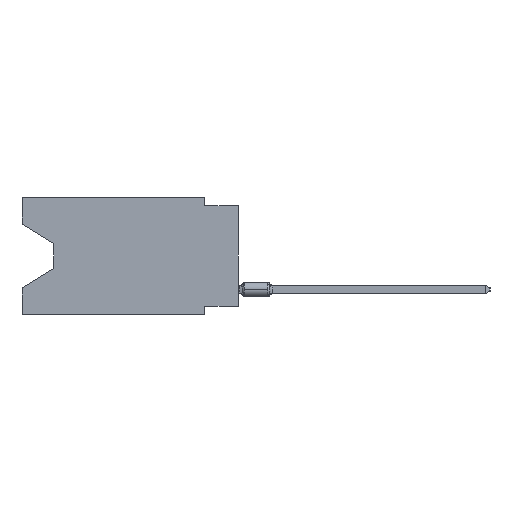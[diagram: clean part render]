
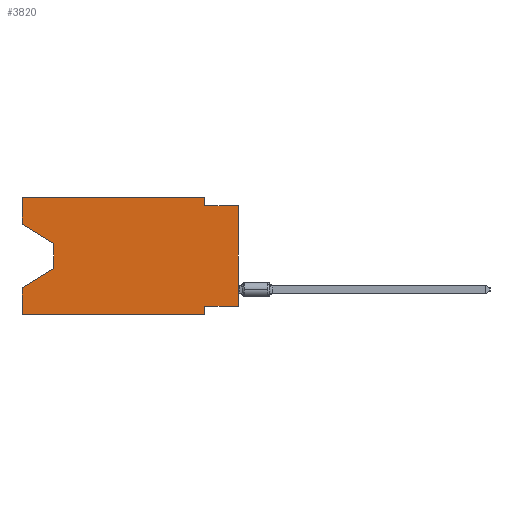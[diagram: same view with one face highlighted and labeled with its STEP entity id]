
A CAD part, left-side view. The second image highlights one B-rep face of the part: STEP entity #3820.
In plain terms, the highlighted planar face has unit normal (-1, 0, 0).
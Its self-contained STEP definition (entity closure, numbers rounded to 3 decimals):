
#179 = EDGE_CURVE ( 'NONE', #42953, #15369, #29749, .T. ) ;
#418 = CARTESIAN_POINT ( 'NONE',  ( 0., 16.383, 0. ) ) ;
#1485 = FACE_OUTER_BOUND ( 'NONE', #47448, .T. ) ;
#3820 = ADVANCED_FACE ( 'NONE', ( #1485 ), #32567, .F. ) ;
#4087 = CARTESIAN_POINT ( 'NONE',  ( 0., 0., 0. ) ) ;
#4166 = EDGE_CURVE ( 'NONE', #33210, #18741, #48302, .T. ) ;
#4488 = CARTESIAN_POINT ( 'NONE',  ( 0., 16.383, -8.89 ) ) ;
#4741 = LINE ( 'NONE', #4488, #46064 ) ;
#6219 = VERTEX_POINT ( 'NONE', #7704 ) ;
#7704 = CARTESIAN_POINT ( 'NONE',  ( 0., 13.97, -3.505 ) ) ;
#7820 = VERTEX_POINT ( 'NONE', #39756 ) ;
#8853 = ORIENTED_EDGE ( 'NONE', *, *, #179, .F. ) ;
#9511 = DIRECTION ( 'NONE',  ( 0., 0., -1. ) ) ;
#10556 = CARTESIAN_POINT ( 'NONE',  ( 0., 16.383, -6.852 ) ) ;
#11437 = LINE ( 'NONE', #26458, #24579 ) ;
#11688 = DIRECTION ( 'NONE',  ( 0., 0.855, -0.519 ) ) ;
#11743 = LINE ( 'NONE', #50327, #17026 ) ;
#11849 = DIRECTION ( 'NONE',  ( 0., 0., 1. ) ) ;
#12112 = LINE ( 'NONE', #4087, #30921 ) ;
#12855 = DIRECTION ( 'NONE',  ( 0., 0., 1. ) ) ;
#14601 = VERTEX_POINT ( 'NONE', #17932 ) ;
#15369 = VERTEX_POINT ( 'NONE', #10556 ) ;
#15539 = EDGE_CURVE ( 'NONE', #6219, #26344, #21351, .T. ) ;
#15604 = DIRECTION ( 'NONE',  ( 0., 0., -1. ) ) ;
#16050 = VERTEX_POINT ( 'NONE', #39013 ) ;
#16078 = CARTESIAN_POINT ( 'NONE',  ( 0., 16.383, 0. ) ) ;
#17026 = VECTOR ( 'NONE', #19267, 1000. ) ;
#17220 = VECTOR ( 'NONE', #17232, 1000. ) ;
#17232 = DIRECTION ( 'NONE',  ( 0., 0., -1. ) ) ;
#17508 = DIRECTION ( 'NONE',  ( 0., -1., 0. ) ) ;
#17626 = DIRECTION ( 'NONE',  ( 0., 0., 1. ) ) ;
#17932 = CARTESIAN_POINT ( 'NONE',  ( 0., 2.54, 0. ) ) ;
#17986 = CARTESIAN_POINT ( 'NONE',  ( 0., 13.97, -3.505 ) ) ;
#18097 = ORIENTED_EDGE ( 'NONE', *, *, #31018, .F. ) ;
#18244 = VERTEX_POINT ( 'NONE', #18737 ) ;
#18737 = CARTESIAN_POINT ( 'NONE',  ( 0., 2.54, -0.635 ) ) ;
#18741 = VERTEX_POINT ( 'NONE', #16078 ) ;
#19163 = ORIENTED_EDGE ( 'NONE', *, *, #27873, .T. ) ;
#19255 = ORIENTED_EDGE ( 'NONE', *, *, #4166, .F. ) ;
#19267 = DIRECTION ( 'NONE',  ( 0., 0., -1. ) ) ;
#19990 = LINE ( 'NONE', #27732, #20601 ) ;
#20547 = DIRECTION ( 'NONE',  ( 0., -1., 0. ) ) ;
#20601 = VECTOR ( 'NONE', #11688, 1000. ) ;
#20701 = CARTESIAN_POINT ( 'NONE',  ( 0., 13.97, -5.385 ) ) ;
#21122 = EDGE_CURVE ( 'NONE', #16050, #7820, #21541, .T. ) ;
#21351 = LINE ( 'NONE', #17986, #17220 ) ;
#21541 = LINE ( 'NONE', #33424, #38347 ) ;
#21878 = EDGE_CURVE ( 'NONE', #18741, #14601, #48809, .T. ) ;
#22906 = EDGE_CURVE ( 'NONE', #18244, #32855, #23531, .T. ) ;
#23531 = LINE ( 'NONE', #27405, #33447 ) ;
#23765 = VECTOR ( 'NONE', #28830, 1000. ) ;
#24295 = DIRECTION ( 'NONE',  ( 1., 0., 0. ) ) ;
#24549 = CARTESIAN_POINT ( 'NONE',  ( 0., 16.383, 0. ) ) ;
#24563 = ORIENTED_EDGE ( 'NONE', *, *, #22906, .F. ) ;
#24579 = VECTOR ( 'NONE', #15604, 1000. ) ;
#25353 = VECTOR ( 'NONE', #12855, 1000. ) ;
#25625 = CARTESIAN_POINT ( 'NONE',  ( 0., 16.383, 0. ) ) ;
#26344 = VERTEX_POINT ( 'NONE', #20701 ) ;
#26458 = CARTESIAN_POINT ( 'NONE',  ( 0., 2.54, 0. ) ) ;
#27405 = CARTESIAN_POINT ( 'NONE',  ( 0., 0., -0.635 ) ) ;
#27732 = CARTESIAN_POINT ( 'NONE',  ( 0., 13.97, -5.385 ) ) ;
#27873 = EDGE_CURVE ( 'NONE', #16050, #32855, #12112, .T. ) ;
#28830 = DIRECTION ( 'NONE',  ( 0., -0.855, -0.519 ) ) ;
#29378 = CARTESIAN_POINT ( 'NONE',  ( 0., 16.383, 0. ) ) ;
#29749 = LINE ( 'NONE', #25625, #30887 ) ;
#30037 = DIRECTION ( 'NONE',  ( 0., 1., 0. ) ) ;
#30326 = AXIS2_PLACEMENT_3D ( 'NONE', #24549, #24295, #9511 ) ;
#30887 = VECTOR ( 'NONE', #17626, 1000. ) ;
#30921 = VECTOR ( 'NONE', #11849, 1000. ) ;
#31018 = EDGE_CURVE ( 'NONE', #7820, #45410, #11743, .T. ) ;
#32070 = DIRECTION ( 'NONE',  ( 0., -1., 0. ) ) ;
#32276 = EDGE_CURVE ( 'NONE', #33210, #6219, #43863, .T. ) ;
#32545 = EDGE_CURVE ( 'NONE', #14601, #18244, #11437, .T. ) ;
#32567 = PLANE ( 'NONE',  #30326 ) ;
#32656 = ORIENTED_EDGE ( 'NONE', *, *, #21878, .F. ) ;
#32855 = VERTEX_POINT ( 'NONE', #50430 ) ;
#33210 = VERTEX_POINT ( 'NONE', #44287 ) ;
#33424 = CARTESIAN_POINT ( 'NONE',  ( 0., 0., -8.255 ) ) ;
#33447 = VECTOR ( 'NONE', #32070, 1000. ) ;
#34300 = EDGE_CURVE ( 'NONE', #26344, #15369, #19990, .T. ) ;
#36122 = CARTESIAN_POINT ( 'NONE',  ( 0., 16.383, -8.89 ) ) ;
#38347 = VECTOR ( 'NONE', #30037, 1000. ) ;
#39013 = CARTESIAN_POINT ( 'NONE',  ( 0., 0., -8.255 ) ) ;
#39719 = ORIENTED_EDGE ( 'NONE', *, *, #21122, .F. ) ;
#39756 = CARTESIAN_POINT ( 'NONE',  ( 0., 2.54, -8.255 ) ) ;
#39958 = VECTOR ( 'NONE', #17508, 1000. ) ;
#42953 = VERTEX_POINT ( 'NONE', #36122 ) ;
#43863 = LINE ( 'NONE', #47736, #23765 ) ;
#44030 = CARTESIAN_POINT ( 'NONE',  ( 0., 2.54, -8.89 ) ) ;
#44287 = CARTESIAN_POINT ( 'NONE',  ( 0., 16.383, -2.038 ) ) ;
#44925 = EDGE_CURVE ( 'NONE', #42953, #45410, #4741, .T. ) ;
#45410 = VERTEX_POINT ( 'NONE', #44030 ) ;
#46064 = VECTOR ( 'NONE', #20547, 1000. ) ;
#46137 = ORIENTED_EDGE ( 'NONE', *, *, #34300, .T. ) ;
#47448 = EDGE_LOOP ( 'NONE', ( #48021, #48893, #46137, #8853, #47684, #18097, #39719, #19163, #24563, #48790, #32656, #19255 ) ) ;
#47684 = ORIENTED_EDGE ( 'NONE', *, *, #44925, .T. ) ;
#47736 = CARTESIAN_POINT ( 'NONE',  ( 0., 16.383, -2.038 ) ) ;
#48021 = ORIENTED_EDGE ( 'NONE', *, *, #32276, .T. ) ;
#48302 = LINE ( 'NONE', #418, #25353 ) ;
#48790 = ORIENTED_EDGE ( 'NONE', *, *, #32545, .F. ) ;
#48809 = LINE ( 'NONE', #29378, #39958 ) ;
#48893 = ORIENTED_EDGE ( 'NONE', *, *, #15539, .T. ) ;
#50327 = CARTESIAN_POINT ( 'NONE',  ( 0., 2.54, -8.89 ) ) ;
#50430 = CARTESIAN_POINT ( 'NONE',  ( 0., 0., -0.635 ) ) ;
